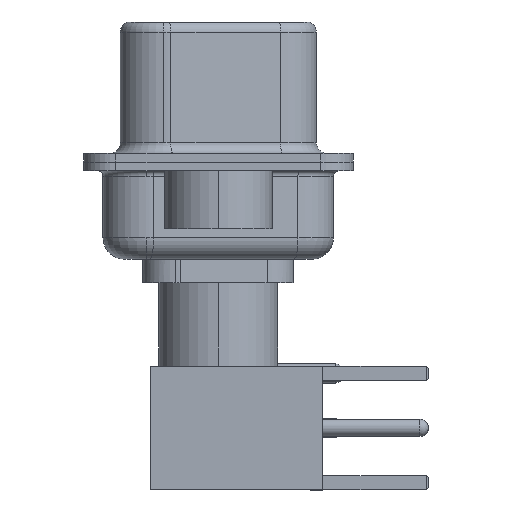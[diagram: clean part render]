
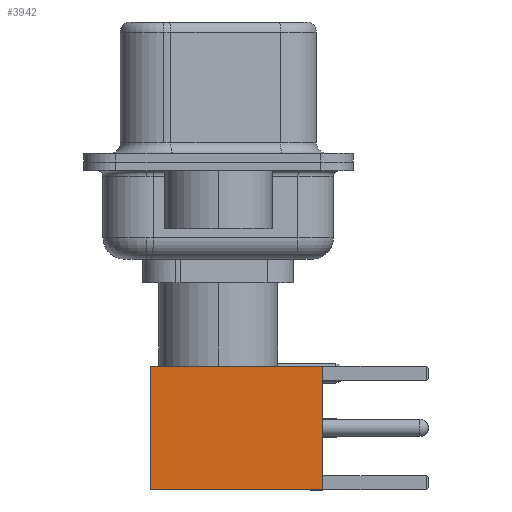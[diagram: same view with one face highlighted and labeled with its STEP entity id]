
A CAD part, left-side view. The second image highlights one B-rep face of the part: STEP entity #3942.
In plain terms, the highlighted face is planar.
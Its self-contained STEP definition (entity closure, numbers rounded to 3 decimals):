
#69 = DIRECTION ( 'NONE',  ( 0., 0., 1. ) ) ;
#3942 = ADVANCED_FACE ( 'NONE', ( #10156 ), #19729, .T. ) ;
#4482 = CARTESIAN_POINT ( 'NONE',  ( 0., 2.875, 0. ) ) ;
#5284 = VERTEX_POINT ( 'NONE', #7888 ) ;
#6026 = CARTESIAN_POINT ( 'NONE',  ( 2.875, 2.875, 0. ) ) ;
#6090 = LINE ( 'NONE', #8391, #21192 ) ;
#6729 = EDGE_CURVE ( 'NONE', #5284, #19261, #9619, .T. ) ;
#7888 = CARTESIAN_POINT ( 'NONE',  ( 2.875, 2.875, 8. ) ) ;
#8391 = CARTESIAN_POINT ( 'NONE',  ( 2.875, 2.875, 0. ) ) ;
#8418 = LINE ( 'NONE', #4482, #15860 ) ;
#8612 = ORIENTED_EDGE ( 'NONE', *, *, #6729, .F. ) ;
#8846 = VERTEX_POINT ( 'NONE', #13616 ) ;
#9619 = LINE ( 'NONE', #12042, #11363 ) ;
#10156 = FACE_OUTER_BOUND ( 'NONE', #19663, .T. ) ;
#11363 = VECTOR ( 'NONE', #17404, 1000. ) ;
#11412 = ORIENTED_EDGE ( 'NONE', *, *, #20503, .F. ) ;
#12042 = CARTESIAN_POINT ( 'NONE',  ( 0., 2.875, 8. ) ) ;
#12803 = ORIENTED_EDGE ( 'NONE', *, *, #22252, .T. ) ;
#13616 = CARTESIAN_POINT ( 'NONE',  ( -2.875, 2.875, 0. ) ) ;
#14661 = DIRECTION ( 'NONE',  ( 0., 0., -1. ) ) ;
#15036 = CARTESIAN_POINT ( 'NONE',  ( -2.875, 2.875, 8. ) ) ;
#15757 = DIRECTION ( 'NONE',  ( 0., 1., 0. ) ) ;
#15860 = VECTOR ( 'NONE', #21836, 1000. ) ;
#16283 = VECTOR ( 'NONE', #14661, 1000. ) ;
#17404 = DIRECTION ( 'NONE',  ( -1., 0., 0. ) ) ;
#17971 = DIRECTION ( 'NONE',  ( 0., 0., -1. ) ) ;
#18634 = LINE ( 'NONE', #18893, #16283 ) ;
#18893 = CARTESIAN_POINT ( 'NONE',  ( -2.875, 2.875, 0. ) ) ;
#19261 = VERTEX_POINT ( 'NONE', #15036 ) ;
#19604 = CARTESIAN_POINT ( 'NONE',  ( 2.875, 2.875, 0. ) ) ;
#19663 = EDGE_LOOP ( 'NONE', ( #12803, #24361, #11412, #8612 ) ) ;
#19729 = PLANE ( 'NONE',  #25187 ) ;
#20503 = EDGE_CURVE ( 'NONE', #19261, #8846, #18634, .T. ) ;
#21192 = VECTOR ( 'NONE', #17971, 1000. ) ;
#21825 = EDGE_CURVE ( 'NONE', #23241, #8846, #8418, .T. ) ;
#21836 = DIRECTION ( 'NONE',  ( -1., 0., 0. ) ) ;
#22252 = EDGE_CURVE ( 'NONE', #5284, #23241, #6090, .T. ) ;
#23241 = VERTEX_POINT ( 'NONE', #6026 ) ;
#24361 = ORIENTED_EDGE ( 'NONE', *, *, #21825, .T. ) ;
#25187 = AXIS2_PLACEMENT_3D ( 'NONE', #19604, #15757, #69 ) ;
